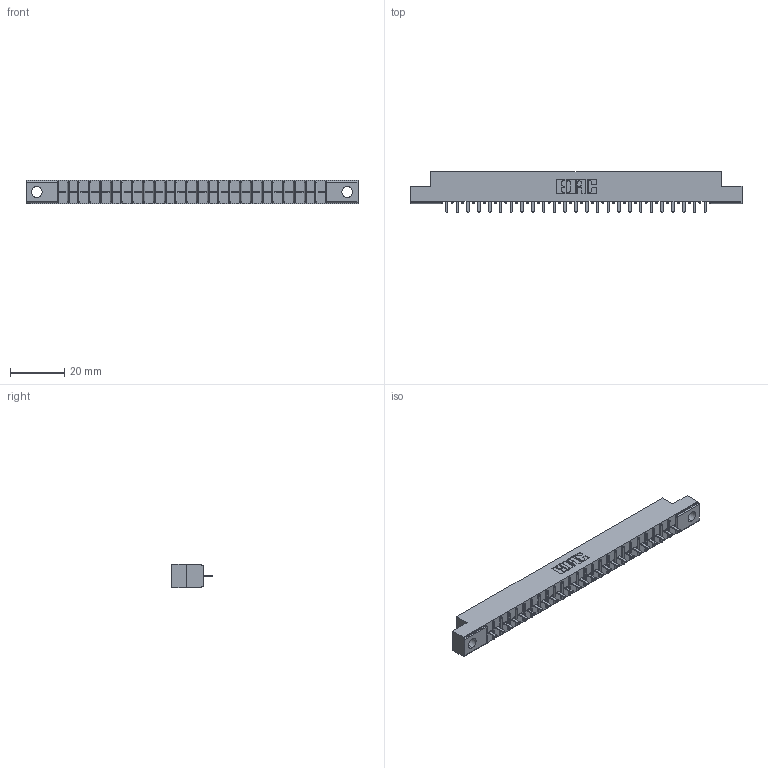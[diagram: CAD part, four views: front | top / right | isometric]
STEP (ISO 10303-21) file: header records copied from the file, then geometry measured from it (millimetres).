
FILE_DESCRIPTION (( 'STEP AP203' ), '1' );
FILE_NAME ('316-025-421-104.STEP', '2020-09-22T22:06:51', ( '' ), ( '' ), 'SwSTEP 2.0', 'SolidWorks 2020', '' );
FILE_SCHEMA (( 'CONFIG_CONTROL_DESIGN' ));
Length unit declared in the file: inch
Products named in the file (3): 306 Part_.156 Dia; 306-290-001_121; 316-025-421-104
Assembly tree (26 placements, depth 2):
  316-025-421-104
    306 Part_.156 Dia
    306-290-001_121  x25
Bounding box: 122.07 x 14.88 x 8.71 mm (x, y, z)
Volume: 8227.9 mm3; surface area: 11939.4 mm2
Topology: 26 solids, 26 shells, 1880 faces, 5277 edges, 3382 vertices
Faces by surface type: plane 1257, cylinder 523, sphere 100
Entity records: 25890 total; most frequent: CARTESIAN_POINT 4348, ORIENTED_EDGE 4306, DIRECTION 4281, EDGE_CURVE 2153, VECTOR 1683, LINE 1683, VERTEX_POINT 1366, AXIS2_PLACEMENT_3D 1299
